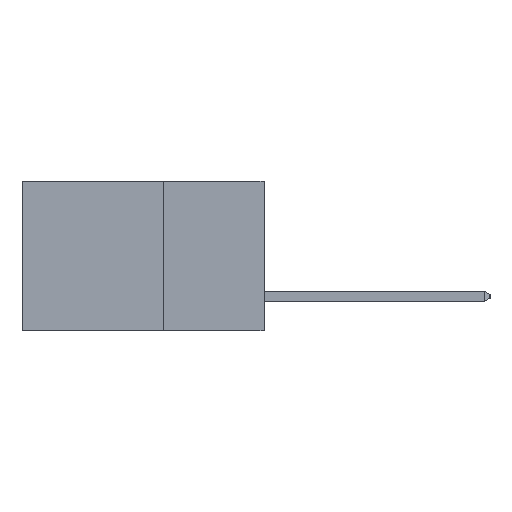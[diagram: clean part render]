
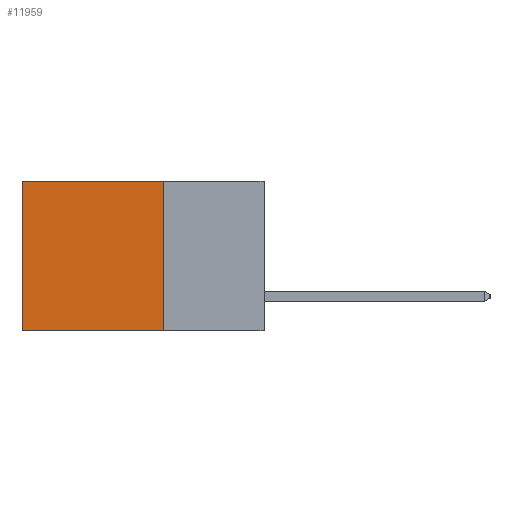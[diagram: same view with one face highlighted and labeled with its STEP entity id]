
A CAD part, left-side view. The second image highlights one B-rep face of the part: STEP entity #11959.
In plain terms, the highlighted planar face has unit normal (-1, 0, 0).
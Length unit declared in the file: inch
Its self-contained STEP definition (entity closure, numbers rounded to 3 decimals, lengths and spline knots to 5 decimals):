
#10 = VERTEX_POINT ( 'NONE', #10267 ) ;
#423 = DIRECTION ( 'NONE',  ( 0., 1., 0. ) ) ;
#475 = CARTESIAN_POINT ( 'NONE',  ( 0.2615, 0.6, 0. ) ) ;
#488 = LINE ( 'NONE', #583, #10840 ) ;
#583 = CARTESIAN_POINT ( 'NONE',  ( 0.2615, 0.6, -0.37 ) ) ;
#656 = EDGE_CURVE ( 'NONE', #3757, #10, #9319, .T. ) ;
#745 = PLANE ( 'NONE',  #5875 ) ;
#1942 = VECTOR ( 'NONE', #423, 39.37008 ) ;
#2034 = ORIENTED_EDGE ( 'NONE', *, *, #5069, .T. ) ;
#2049 = ORIENTED_EDGE ( 'NONE', *, *, #656, .F. ) ;
#2143 = ORIENTED_EDGE ( 'NONE', *, *, #3029, .F. ) ;
#2157 = ORIENTED_EDGE ( 'NONE', *, *, #10186, .T. ) ;
#2540 = CARTESIAN_POINT ( 'NONE',  ( 0.2615, 0.25, -0.37 ) ) ;
#3029 = EDGE_CURVE ( 'NONE', #6628, #3757, #8836, .T. ) ;
#3631 = EDGE_LOOP ( 'NONE', ( #2034, #2049, #2143, #2157 ) ) ;
#3757 = VERTEX_POINT ( 'NONE', #11348 ) ;
#4320 = CARTESIAN_POINT ( 'NONE',  ( 0.2615, 0.25, -0.37 ) ) ;
#4913 = CARTESIAN_POINT ( 'NONE',  ( 0.2615, 0.25, 0. ) ) ;
#5069 = EDGE_CURVE ( 'NONE', #6766, #10, #488, .T. ) ;
#5448 = DIRECTION ( 'NONE',  ( 0., 0., -1. ) ) ;
#5875 = AXIS2_PLACEMENT_3D ( 'NONE', #4320, #10749, #5448 ) ;
#6628 = VERTEX_POINT ( 'NONE', #4913 ) ;
#6766 = VERTEX_POINT ( 'NONE', #475 ) ;
#6968 = CARTESIAN_POINT ( 'NONE',  ( 0.2615, 0.25, 0. ) ) ;
#6987 = VECTOR ( 'NONE', #8774, 39.37008 ) ;
#7413 = FACE_OUTER_BOUND ( 'NONE', #3631, .T. ) ;
#8774 = DIRECTION ( 'NONE',  ( 0., 1., 0. ) ) ;
#8836 = LINE ( 'NONE', #9872, #9092 ) ;
#8952 = DIRECTION ( 'NONE',  ( 0., 0., -1. ) ) ;
#9092 = VECTOR ( 'NONE', #9553, 39.37008 ) ;
#9319 = LINE ( 'NONE', #2540, #6987 ) ;
#9553 = DIRECTION ( 'NONE',  ( 0., 0., -1. ) ) ;
#9872 = CARTESIAN_POINT ( 'NONE',  ( 0.2615, 0.25, -0.37 ) ) ;
#10186 = EDGE_CURVE ( 'NONE', #6628, #6766, #12354, .T. ) ;
#10267 = CARTESIAN_POINT ( 'NONE',  ( 0.2615, 0.6, -0.37 ) ) ;
#10749 = DIRECTION ( 'NONE',  ( 1., 0., 0. ) ) ;
#10840 = VECTOR ( 'NONE', #8952, 39.37008 ) ;
#11348 = CARTESIAN_POINT ( 'NONE',  ( 0.2615, 0.25, -0.37 ) ) ;
#11959 = ADVANCED_FACE ( 'NONE', ( #7413 ), #745, .F. ) ;
#12354 = LINE ( 'NONE', #6968, #1942 ) ;
